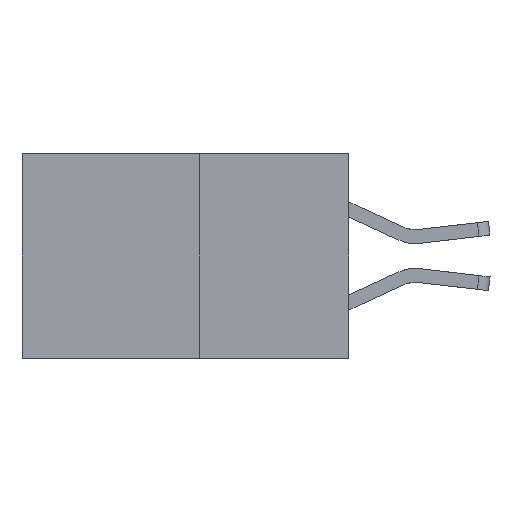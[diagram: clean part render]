
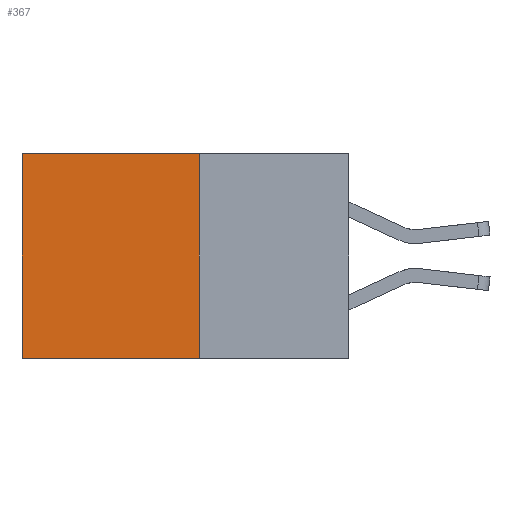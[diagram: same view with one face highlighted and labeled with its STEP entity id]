
A CAD part, left-side view. The second image highlights one B-rep face of the part: STEP entity #367.
In plain terms, the highlighted planar face has unit normal (-1, 0, 0).
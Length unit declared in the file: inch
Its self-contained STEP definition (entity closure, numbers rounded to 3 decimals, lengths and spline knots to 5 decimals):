
#367 = ADVANCED_FACE ( 'NONE', ( #1902 ), #8353, .F. ) ;
#814 = VERTEX_POINT ( 'NONE', #7604 ) ;
#1286 = LINE ( 'NONE', #8284, #4678 ) ;
#1380 = VERTEX_POINT ( 'NONE', #2841 ) ;
#1681 = EDGE_CURVE ( 'NONE', #7800, #5236, #5637, .T. ) ;
#1863 = LINE ( 'NONE', #3406, #3882 ) ;
#1902 = FACE_OUTER_BOUND ( 'NONE', #2783, .T. ) ;
#1912 = ORIENTED_EDGE ( 'NONE', *, *, #4563, .T. ) ;
#2073 = CARTESIAN_POINT ( 'NONE',  ( 0.277, 0.27, -0.37 ) ) ;
#2783 = EDGE_LOOP ( 'NONE', ( #1912, #4304, #6062, #7919 ) ) ;
#2841 = CARTESIAN_POINT ( 'NONE',  ( 0.277, 0.59, 0. ) ) ;
#3377 = DIRECTION ( 'NONE',  ( 0., 0., -1. ) ) ;
#3406 = CARTESIAN_POINT ( 'NONE',  ( 0.277, 0.59, -0.37 ) ) ;
#3410 = VECTOR ( 'NONE', #5179, 39.37008 ) ;
#3810 = VECTOR ( 'NONE', #3886, 39.37008 ) ;
#3882 = VECTOR ( 'NONE', #3377, 39.37008 ) ;
#3886 = DIRECTION ( 'NONE',  ( 0., 0., -1. ) ) ;
#4304 = ORIENTED_EDGE ( 'NONE', *, *, #6446, .F. ) ;
#4488 = CARTESIAN_POINT ( 'NONE',  ( 0.277, 0.27, 0. ) ) ;
#4563 = EDGE_CURVE ( 'NONE', #1380, #814, #1863, .T. ) ;
#4678 = VECTOR ( 'NONE', #7521, 39.37008 ) ;
#5179 = DIRECTION ( 'NONE',  ( 0., 1., 0. ) ) ;
#5185 = CARTESIAN_POINT ( 'NONE',  ( 0.277, 0.27, -0.37 ) ) ;
#5236 = VERTEX_POINT ( 'NONE', #2073 ) ;
#5637 = LINE ( 'NONE', #7598, #3810 ) ;
#6062 = ORIENTED_EDGE ( 'NONE', *, *, #1681, .F. ) ;
#6446 = EDGE_CURVE ( 'NONE', #5236, #814, #1286, .T. ) ;
#7004 = AXIS2_PLACEMENT_3D ( 'NONE', #5185, #8332, #7132 ) ;
#7132 = DIRECTION ( 'NONE',  ( 0., 0., -1. ) ) ;
#7253 = LINE ( 'NONE', #4488, #3410 ) ;
#7521 = DIRECTION ( 'NONE',  ( 0., 1., 0. ) ) ;
#7598 = CARTESIAN_POINT ( 'NONE',  ( 0.277, 0.27, -0.37 ) ) ;
#7604 = CARTESIAN_POINT ( 'NONE',  ( 0.277, 0.59, -0.37 ) ) ;
#7800 = VERTEX_POINT ( 'NONE', #8574 ) ;
#7919 = ORIENTED_EDGE ( 'NONE', *, *, #8172, .T. ) ;
#8172 = EDGE_CURVE ( 'NONE', #7800, #1380, #7253, .T. ) ;
#8284 = CARTESIAN_POINT ( 'NONE',  ( 0.277, 0.27, -0.37 ) ) ;
#8332 = DIRECTION ( 'NONE',  ( 1., 0., 0. ) ) ;
#8353 = PLANE ( 'NONE',  #7004 ) ;
#8574 = CARTESIAN_POINT ( 'NONE',  ( 0.277, 0.27, 0. ) ) ;
